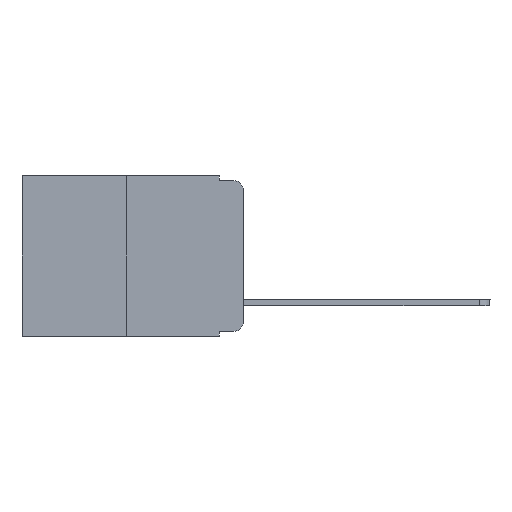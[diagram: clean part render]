
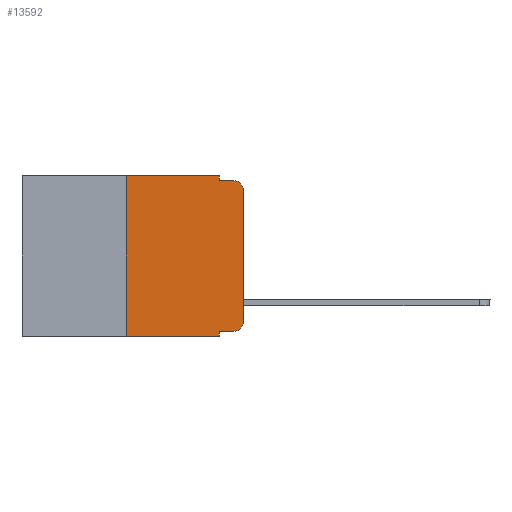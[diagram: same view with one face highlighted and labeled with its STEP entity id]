
A CAD part, left-side view. The second image highlights one B-rep face of the part: STEP entity #13592.
In plain terms, the highlighted planar face has unit normal (-1, 0, 0).
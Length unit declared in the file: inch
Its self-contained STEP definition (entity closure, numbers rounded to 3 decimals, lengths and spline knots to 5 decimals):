
#57 = ORIENTED_EDGE ( 'NONE', *, *, #10432, .T. ) ;
#221 = CARTESIAN_POINT ( 'NONE',  ( 0., 0.25, 0. ) ) ;
#341 = VERTEX_POINT ( 'NONE', #11248 ) ;
#535 = VECTOR ( 'NONE', #10635, 39.37008 ) ;
#660 = LINE ( 'NONE', #1686, #8420 ) ;
#1058 = AXIS2_PLACEMENT_3D ( 'NONE', #2287, #6744, #10078 ) ;
#1079 = EDGE_CURVE ( 'NONE', #341, #8436, #3763, .T. ) ;
#1101 = VERTEX_POINT ( 'NONE', #8204 ) ;
#1137 = CARTESIAN_POINT ( 'NONE',  ( 0., 0.25, -0.343 ) ) ;
#1429 = ORIENTED_EDGE ( 'NONE', *, *, #2394, .F. ) ;
#1487 = AXIS2_PLACEMENT_3D ( 'NONE', #3614, #4496, #8055 ) ;
#1640 = ORIENTED_EDGE ( 'NONE', *, *, #4382, .F. ) ;
#1686 = CARTESIAN_POINT ( 'NONE',  ( 0., 0.25, 0. ) ) ;
#1704 = VERTEX_POINT ( 'NONE', #9570 ) ;
#1965 = LINE ( 'NONE', #5331, #3500 ) ;
#2104 = LINE ( 'NONE', #5245, #535 ) ;
#2144 = EDGE_CURVE ( 'NONE', #9023, #3706, #660, .T. ) ;
#2287 = CARTESIAN_POINT ( 'NONE',  ( 0., 0.473, 0. ) ) ;
#2379 = EDGE_CURVE ( 'NONE', #9023, #3377, #1965, .T. ) ;
#2394 = EDGE_CURVE ( 'NONE', #3706, #7467, #4664, .T. ) ;
#2681 = CARTESIAN_POINT ( 'NONE',  ( 0., 0.051, -0.333 ) ) ;
#2690 = VERTEX_POINT ( 'NONE', #2979 ) ;
#2721 = VECTOR ( 'NONE', #2735, 39.37008 ) ;
#2735 = DIRECTION ( 'NONE',  ( 0., 0., -1. ) ) ;
#2748 = VECTOR ( 'NONE', #3563, 39.37008 ) ;
#2831 = VECTOR ( 'NONE', #5656, 39.37008 ) ;
#2939 = EDGE_CURVE ( 'NONE', #2690, #11958, #12418, .T. ) ;
#2979 = CARTESIAN_POINT ( 'NONE',  ( 0., 0.02, -0.333 ) ) ;
#3275 = DIRECTION ( 'NONE',  ( 0., 0., -1. ) ) ;
#3377 = VERTEX_POINT ( 'NONE', #11234 ) ;
#3500 = VECTOR ( 'NONE', #13532, 39.37008 ) ;
#3563 = DIRECTION ( 'NONE',  ( 0., -1., 0. ) ) ;
#3564 = ORIENTED_EDGE ( 'NONE', *, *, #2379, .T. ) ;
#3602 = LINE ( 'NONE', #13647, #2831 ) ;
#3614 = CARTESIAN_POINT ( 'NONE',  ( 0., 0.02, -0.313 ) ) ;
#3706 = VERTEX_POINT ( 'NONE', #221 ) ;
#3763 = LINE ( 'NONE', #10043, #7253 ) ;
#3809 = VECTOR ( 'NONE', #10542, 39.37008 ) ;
#4107 = CARTESIAN_POINT ( 'NONE',  ( 0., 0.051, 0. ) ) ;
#4382 = EDGE_CURVE ( 'NONE', #1704, #3377, #13936, .T. ) ;
#4496 = DIRECTION ( 'NONE',  ( -1., 0., 0. ) ) ;
#4630 = ORIENTED_EDGE ( 'NONE', *, *, #1079, .F. ) ;
#4664 = LINE ( 'NONE', #9025, #2748 ) ;
#5015 = LINE ( 'NONE', #2681, #3809 ) ;
#5245 = CARTESIAN_POINT ( 'NONE',  ( 0., 0.051, 0. ) ) ;
#5331 = CARTESIAN_POINT ( 'NONE',  ( 0., 0.473, -0.343 ) ) ;
#5656 = DIRECTION ( 'NONE',  ( 0., 0., 1. ) ) ;
#5747 = CARTESIAN_POINT ( 'NONE',  ( 0., 0.02, -0.03 ) ) ;
#5942 = CARTESIAN_POINT ( 'NONE',  ( 0., 0., -0.313 ) ) ;
#6744 = DIRECTION ( 'NONE',  ( 1., 0., 0. ) ) ;
#7253 = VECTOR ( 'NONE', #8883, 39.37008 ) ;
#7467 = VERTEX_POINT ( 'NONE', #4107 ) ;
#7818 = FACE_OUTER_BOUND ( 'NONE', #11870, .T. ) ;
#7822 = EDGE_CURVE ( 'NONE', #11958, #1101, #3602, .T. ) ;
#7891 = PLANE ( 'NONE',  #1058 ) ;
#8055 = DIRECTION ( 'NONE',  ( 0., 0., -1. ) ) ;
#8204 = CARTESIAN_POINT ( 'NONE',  ( 0., 0., -0.03 ) ) ;
#8420 = VECTOR ( 'NONE', #10428, 39.37008 ) ;
#8436 = VERTEX_POINT ( 'NONE', #10435 ) ;
#8799 = ORIENTED_EDGE ( 'NONE', *, *, #10325, .F. ) ;
#8883 = DIRECTION ( 'NONE',  ( 0., -1., 0. ) ) ;
#8943 = DIRECTION ( 'NONE',  ( -1., 0., 0. ) ) ;
#9023 = VERTEX_POINT ( 'NONE', #1137 ) ;
#9025 = CARTESIAN_POINT ( 'NONE',  ( 0., 0.473, 0. ) ) ;
#9374 = CIRCLE ( 'NONE', #10077, 0.02 ) ;
#9570 = CARTESIAN_POINT ( 'NONE',  ( 0., 0.051, -0.333 ) ) ;
#10043 = CARTESIAN_POINT ( 'NONE',  ( 0., 0.051, -0.01 ) ) ;
#10077 = AXIS2_PLACEMENT_3D ( 'NONE', #5747, #8943, #3275 ) ;
#10078 = DIRECTION ( 'NONE',  ( 0., 0., -1. ) ) ;
#10325 = EDGE_CURVE ( 'NONE', #7467, #341, #2104, .T. ) ;
#10428 = DIRECTION ( 'NONE',  ( 0., 0., 1. ) ) ;
#10432 = EDGE_CURVE ( 'NONE', #1101, #8436, #9374, .T. ) ;
#10435 = CARTESIAN_POINT ( 'NONE',  ( 0., 0.02, -0.01 ) ) ;
#10542 = DIRECTION ( 'NONE',  ( 0., -1., 0. ) ) ;
#10610 = EDGE_CURVE ( 'NONE', #1704, #2690, #5015, .T. ) ;
#10635 = DIRECTION ( 'NONE',  ( 0., 0., -1. ) ) ;
#11234 = CARTESIAN_POINT ( 'NONE',  ( 0., 0.051, -0.343 ) ) ;
#11248 = CARTESIAN_POINT ( 'NONE',  ( 0., 0.051, -0.01 ) ) ;
#11361 = ORIENTED_EDGE ( 'NONE', *, *, #10610, .T. ) ;
#11870 = EDGE_LOOP ( 'NONE', ( #11888, #57, #4630, #8799, #1429, #13245, #3564, #1640, #11361, #14260 ) ) ;
#11888 = ORIENTED_EDGE ( 'NONE', *, *, #7822, .T. ) ;
#11958 = VERTEX_POINT ( 'NONE', #5942 ) ;
#12418 = CIRCLE ( 'NONE', #1487, 0.02 ) ;
#13245 = ORIENTED_EDGE ( 'NONE', *, *, #2144, .F. ) ;
#13532 = DIRECTION ( 'NONE',  ( 0., -1., 0. ) ) ;
#13592 = ADVANCED_FACE ( 'NONE', ( #7818 ), #7891, .F. ) ;
#13647 = CARTESIAN_POINT ( 'NONE',  ( 0., 0., 0. ) ) ;
#13718 = CARTESIAN_POINT ( 'NONE',  ( 0., 0.051, 0. ) ) ;
#13936 = LINE ( 'NONE', #13718, #2721 ) ;
#14260 = ORIENTED_EDGE ( 'NONE', *, *, #2939, .T. ) ;
